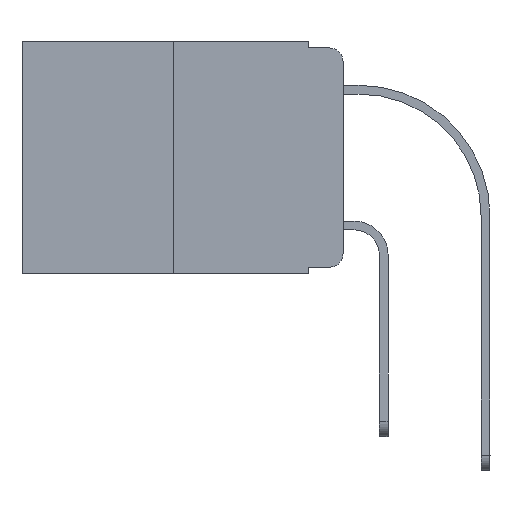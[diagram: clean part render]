
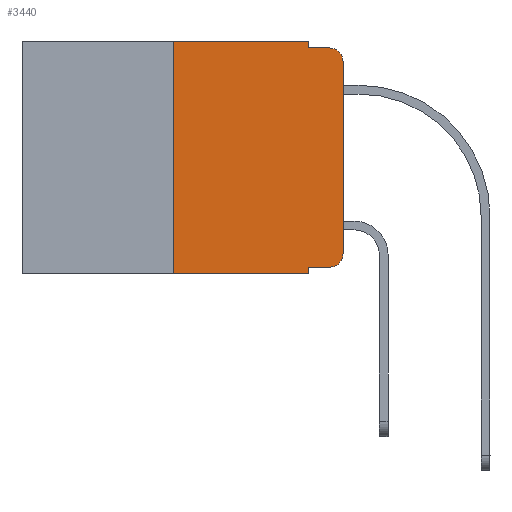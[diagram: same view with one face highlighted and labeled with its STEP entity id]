
A CAD part, left-side view. The second image highlights one B-rep face of the part: STEP entity #3440.
In plain terms, the highlighted planar face has unit normal (-1, 0, 0).
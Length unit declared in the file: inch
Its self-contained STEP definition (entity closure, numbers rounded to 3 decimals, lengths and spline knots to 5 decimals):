
#292 = LINE ( 'NONE', #6192, #15024 ) ;
#545 = CARTESIAN_POINT ( 'NONE',  ( 0., 0.25, -0.343 ) ) ;
#1093 = DIRECTION ( 'NONE',  ( 1., 0., 0. ) ) ;
#1128 = DIRECTION ( 'NONE',  ( 0., -1., 0. ) ) ;
#1214 = AXIS2_PLACEMENT_3D ( 'NONE', #15189, #1093, #2362 ) ;
#1425 = DIRECTION ( 'NONE',  ( 0., 0., -1. ) ) ;
#1548 = EDGE_CURVE ( 'NONE', #3684, #14636, #2791, .T. ) ;
#1559 = CARTESIAN_POINT ( 'NONE',  ( 0., 0., -0.313 ) ) ;
#1819 = LINE ( 'NONE', #1889, #7673 ) ;
#1889 = CARTESIAN_POINT ( 'NONE',  ( 0., 0.473, 0. ) ) ;
#1999 = DIRECTION ( 'NONE',  ( 0., 0., 1. ) ) ;
#2345 = CARTESIAN_POINT ( 'NONE',  ( 0., 0.051, -0.333 ) ) ;
#2362 = DIRECTION ( 'NONE',  ( 0., 0., -1. ) ) ;
#2580 = CARTESIAN_POINT ( 'NONE',  ( 0., 0.25, 0. ) ) ;
#2686 = LINE ( 'NONE', #9966, #3619 ) ;
#2791 = LINE ( 'NONE', #7502, #5197 ) ;
#2863 = DIRECTION ( 'NONE',  ( -1., 0., 0. ) ) ;
#3170 = CARTESIAN_POINT ( 'NONE',  ( 0., 0.25, 0. ) ) ;
#3440 = ADVANCED_FACE ( 'NONE', ( #10510 ), #7078, .F. ) ;
#3582 = LINE ( 'NONE', #13063, #14816 ) ;
#3619 = VECTOR ( 'NONE', #1425, 39.37008 ) ;
#3672 = DIRECTION ( 'NONE',  ( 0., -1., 0. ) ) ;
#3673 = CARTESIAN_POINT ( 'NONE',  ( 0., 0., 0. ) ) ;
#3684 = VERTEX_POINT ( 'NONE', #6906 ) ;
#4289 = DIRECTION ( 'NONE',  ( 0., -1., 0. ) ) ;
#4791 = ORIENTED_EDGE ( 'NONE', *, *, #6279, .F. ) ;
#4865 = CARTESIAN_POINT ( 'NONE',  ( 0., 0., -0.03 ) ) ;
#4951 = VECTOR ( 'NONE', #4289, 39.37008 ) ;
#5155 = ORIENTED_EDGE ( 'NONE', *, *, #12296, .T. ) ;
#5195 = CARTESIAN_POINT ( 'NONE',  ( 0., 0.02, -0.313 ) ) ;
#5197 = VECTOR ( 'NONE', #7581, 39.37008 ) ;
#5592 = VERTEX_POINT ( 'NONE', #2580 ) ;
#5738 = VERTEX_POINT ( 'NONE', #1559 ) ;
#6108 = EDGE_CURVE ( 'NONE', #6924, #7945, #2686, .T. ) ;
#6192 = CARTESIAN_POINT ( 'NONE',  ( 0., 0.051, -0.333 ) ) ;
#6279 = EDGE_CURVE ( 'NONE', #5592, #3684, #1819, .T. ) ;
#6580 = CARTESIAN_POINT ( 'NONE',  ( 0., 0.02, -0.03 ) ) ;
#6620 = DIRECTION ( 'NONE',  ( 0., -1., 0. ) ) ;
#6646 = DIRECTION ( 'NONE',  ( -1., 0., 0. ) ) ;
#6658 = LINE ( 'NONE', #11402, #4951 ) ;
#6722 = DIRECTION ( 'NONE',  ( 0., 0., -1. ) ) ;
#6906 = CARTESIAN_POINT ( 'NONE',  ( 0., 0.051, 0. ) ) ;
#6924 = VERTEX_POINT ( 'NONE', #2345 ) ;
#6967 = CIRCLE ( 'NONE', #9970, 0.02 ) ;
#6976 = LINE ( 'NONE', #3673, #6980 ) ;
#6980 = VECTOR ( 'NONE', #11732, 39.37008 ) ;
#7078 = PLANE ( 'NONE',  #1214 ) ;
#7177 = EDGE_CURVE ( 'NONE', #14636, #13410, #6658, .T. ) ;
#7459 = ORIENTED_EDGE ( 'NONE', *, *, #1548, .F. ) ;
#7502 = CARTESIAN_POINT ( 'NONE',  ( 0., 0.051, 0. ) ) ;
#7543 = ORIENTED_EDGE ( 'NONE', *, *, #8005, .T. ) ;
#7581 = DIRECTION ( 'NONE',  ( 0., 0., -1. ) ) ;
#7673 = VECTOR ( 'NONE', #6620, 39.37008 ) ;
#7945 = VERTEX_POINT ( 'NONE', #8393 ) ;
#8005 = EDGE_CURVE ( 'NONE', #5738, #10729, #6976, .T. ) ;
#8393 = CARTESIAN_POINT ( 'NONE',  ( 0., 0.051, -0.343 ) ) ;
#8751 = EDGE_CURVE ( 'NONE', #10729, #13410, #6967, .T. ) ;
#9135 = LINE ( 'NONE', #3170, #10251 ) ;
#9372 = ORIENTED_EDGE ( 'NONE', *, *, #14979, .T. ) ;
#9966 = CARTESIAN_POINT ( 'NONE',  ( 0., 0.051, 0. ) ) ;
#9970 = AXIS2_PLACEMENT_3D ( 'NONE', #6580, #6646, #6722 ) ;
#10169 = EDGE_LOOP ( 'NONE', ( #7543, #10406, #13174, #7459, #4791, #14926, #5155, #13258, #9372, #14694 ) ) ;
#10251 = VECTOR ( 'NONE', #1999, 39.37008 ) ;
#10406 = ORIENTED_EDGE ( 'NONE', *, *, #8751, .T. ) ;
#10510 = FACE_OUTER_BOUND ( 'NONE', #10169, .T. ) ;
#10729 = VERTEX_POINT ( 'NONE', #4865 ) ;
#11402 = CARTESIAN_POINT ( 'NONE',  ( 0., 0.051, -0.01 ) ) ;
#11732 = DIRECTION ( 'NONE',  ( 0., 0., 1. ) ) ;
#11788 = EDGE_CURVE ( 'NONE', #12842, #5738, #15037, .T. ) ;
#12153 = CARTESIAN_POINT ( 'NONE',  ( 0., 0.02, -0.333 ) ) ;
#12279 = AXIS2_PLACEMENT_3D ( 'NONE', #5195, #2863, #12405 ) ;
#12296 = EDGE_CURVE ( 'NONE', #13395, #7945, #3582, .T. ) ;
#12405 = DIRECTION ( 'NONE',  ( 0., 0., -1. ) ) ;
#12842 = VERTEX_POINT ( 'NONE', #12153 ) ;
#13063 = CARTESIAN_POINT ( 'NONE',  ( 0., 0.473, -0.343 ) ) ;
#13174 = ORIENTED_EDGE ( 'NONE', *, *, #7177, .F. ) ;
#13258 = ORIENTED_EDGE ( 'NONE', *, *, #6108, .F. ) ;
#13395 = VERTEX_POINT ( 'NONE', #545 ) ;
#13410 = VERTEX_POINT ( 'NONE', #13572 ) ;
#13572 = CARTESIAN_POINT ( 'NONE',  ( 0., 0.02, -0.01 ) ) ;
#13793 = CARTESIAN_POINT ( 'NONE',  ( 0., 0.051, -0.01 ) ) ;
#13813 = EDGE_CURVE ( 'NONE', #13395, #5592, #9135, .T. ) ;
#14636 = VERTEX_POINT ( 'NONE', #13793 ) ;
#14694 = ORIENTED_EDGE ( 'NONE', *, *, #11788, .T. ) ;
#14816 = VECTOR ( 'NONE', #1128, 39.37008 ) ;
#14926 = ORIENTED_EDGE ( 'NONE', *, *, #13813, .F. ) ;
#14979 = EDGE_CURVE ( 'NONE', #6924, #12842, #292, .T. ) ;
#15024 = VECTOR ( 'NONE', #3672, 39.37008 ) ;
#15037 = CIRCLE ( 'NONE', #12279, 0.02 ) ;
#15189 = CARTESIAN_POINT ( 'NONE',  ( 0., 0.473, 0. ) ) ;
